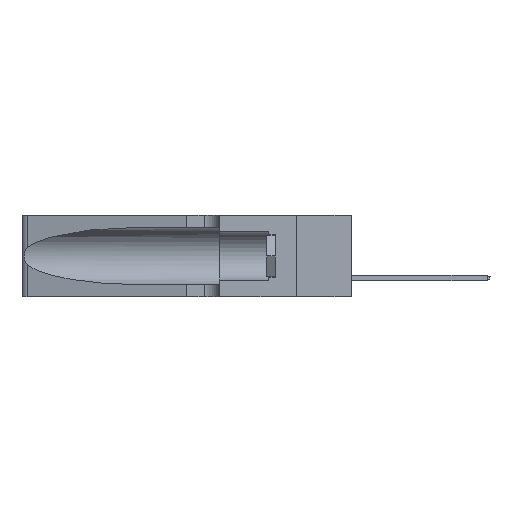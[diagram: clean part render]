
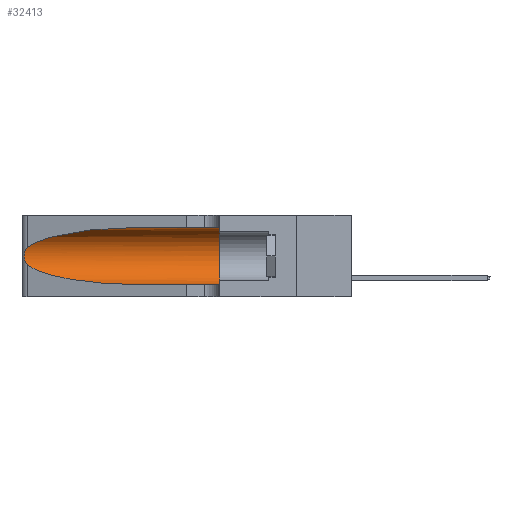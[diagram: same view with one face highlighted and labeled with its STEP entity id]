
A CAD part, left-side view. The second image highlights one B-rep face of the part: STEP entity #32413.
In plain terms, the highlighted cylindrical face has radius 3.308 mm (diameter 6.617 mm), a partial arc.
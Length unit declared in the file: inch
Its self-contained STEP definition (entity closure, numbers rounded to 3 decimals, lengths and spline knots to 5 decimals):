
#82 = CIRCLE ( 'NONE', #31931, 0.13025 ) ;
#206 = VERTEX_POINT ( 'NONE', #14454 ) ;
#1051 = DIRECTION ( 'NONE',  ( 0., -1., 0. ) ) ;
#1223 = CARTESIAN_POINT ( 'NONE',  ( 0.25487, 1.22718, 0.14631 ) ) ;
#1243 = CARTESIAN_POINT ( 'NONE',  ( 0.26075, 1.23896, 0.19203 ) ) ;
#1700 = ORIENTED_EDGE ( 'NONE', *, *, #35580, .T. ) ;
#3316 = EDGE_CURVE ( 'NONE', #7978, #206, #35586, .T. ) ;
#3819 = LINE ( 'NONE', #14539, #11201 ) ;
#4359 = EDGE_CURVE ( 'NONE', #7978, #28881, #15083, .T. ) ;
#5092 = CARTESIAN_POINT ( 'NONE',  ( 0.25856, 1.23593, 0.16098 ) ) ;
#5230 = CARTESIAN_POINT ( 'NONE',  ( 0.1305, 0.72297, 0.31525 ) ) ;
#6283 = CARTESIAN_POINT ( 'NONE',  ( 0.2373, 1.15595, 0.28018 ) ) ;
#6428 = CARTESIAN_POINT ( 'NONE',  ( 0.1305, 0.72297, 0.31525 ) ) ;
#7680 = CARTESIAN_POINT ( 'NONE',  ( 0.1305, 1.61858, 0.185 ) ) ;
#7978 = VERTEX_POINT ( 'NONE', #5230 ) ;
#8002 = CARTESIAN_POINT ( 'NONE',  ( 0.26017, 1.23833, 0.17102 ) ) ;
#8470 = CARTESIAN_POINT ( 'NONE',  ( 0.25487, 1.22718, 0.22369 ) ) ;
#9814 = CARTESIAN_POINT ( 'NONE',  ( 0.1305, 0.35, 0.185 ) ) ;
#10583 = CARTESIAN_POINT ( 'NONE',  ( 0.1305, 0.35, 0.31525 ) ) ;
#10893 = CARTESIAN_POINT ( 'NONE',  ( 0.18966, 0.96281, 0.05475 ) ) ;
#11041 = CARTESIAN_POINT ( 'NONE',  ( 0.1305, 0.72297, 0.05475 ) ) ;
#11070 = CARTESIAN_POINT ( 'NONE',  ( 0.1305, 0.35, 0.05475 ) ) ;
#11201 = VECTOR ( 'NONE', #21382, 39.37008 ) ;
#11645 = ORIENTED_EDGE ( 'NONE', *, *, #4359, .F. ) ;
#12899 = DIRECTION ( 'NONE',  ( 0., 1., 0. ) ) ;
#13308 = CARTESIAN_POINT ( 'NONE',  ( 0.18966, 0.96281, 0.31525 ) ) ;
#13365 = CARTESIAN_POINT ( 'NONE',  ( 0.1305, 0.72297, 0.05475 ) ) ;
#13626 = CARTESIAN_POINT ( 'NONE',  ( 0.1305, 1.61858, 0.31525 ) ) ;
#13646 = EDGE_CURVE ( 'NONE', #206, #31833, #38542, .T. ) ;
#14454 = CARTESIAN_POINT ( 'NONE',  ( 0.25487, 1.22718, 0.22369 ) ) ;
#14539 = CARTESIAN_POINT ( 'NONE',  ( 0.1305, 1.61858, 0.05475 ) ) ;
#14597 = DIRECTION ( 'NONE',  ( 0., 0., -1. ) ) ;
#15083 = LINE ( 'NONE', #13626, #16662 ) ;
#15721 = CYLINDRICAL_SURFACE ( 'NONE', #19944, 0.13025 ) ;
#16662 = VECTOR ( 'NONE', #27362, 39.37008 ) ;
#17734 = EDGE_CURVE ( 'NONE', #28881, #19556, #82, .T. ) ;
#18363 = CARTESIAN_POINT ( 'NONE',  ( 0.25639, 1.23184, 0.21858 ) ) ;
#19556 = VERTEX_POINT ( 'NONE', #11070 ) ;
#19944 = AXIS2_PLACEMENT_3D ( 'NONE', #7680, #1051, #14597 ) ;
#20816 = CARTESIAN_POINT ( 'NONE',  ( 0.2373, 1.15595, 0.08982 ) ) ;
#21382 = DIRECTION ( 'NONE',  ( 0., -1., 0. ) ) ;
#21464 = CARTESIAN_POINT ( 'NONE',  ( 0.26075, 1.23896, 0.178 ) ) ;
#21618 = CARTESIAN_POINT ( 'NONE',  ( 0.25854, 1.2359, 0.20912 ) ) ;
#25204 = ORIENTED_EDGE ( 'NONE', *, *, #3316, .T. ) ;
#25352 = CARTESIAN_POINT ( 'NONE',  ( 0.25555, 1.22994, 0.2215 ) ) ;
#26690 = VERTEX_POINT ( 'NONE', #13365 ) ;
#27362 = DIRECTION ( 'NONE',  ( 0., -1., 0. ) ) ;
#28578 = CARTESIAN_POINT ( 'NONE',  ( 0.25555, 1.22993, 0.14849 ) ) ;
#28733 = CARTESIAN_POINT ( 'NONE',  ( 0.25639, 1.23186, 0.15144 ) ) ;
#28881 = VERTEX_POINT ( 'NONE', #10583 ) ;
#29905 = CARTESIAN_POINT ( 'NONE',  ( 0.25487, 1.22718, 0.22369 ) ) ;
#30506 = ORIENTED_EDGE ( 'NONE', *, *, #37550, .T. ) ;
#31833 = VERTEX_POINT ( 'NONE', #1223 ) ;
#31931 = AXIS2_PLACEMENT_3D ( 'NONE', #9814, #12899, #33477 ) ;
#32413 = ADVANCED_FACE ( 'NONE', ( #40983 ), #15721, .F. ) ;
#33477 = DIRECTION ( 'NONE',  ( 0., 0., 1. ) ) ;
#33951 = EDGE_LOOP ( 'NONE', ( #25204, #42934, #30506, #1700, #38205, #11645 ) ) ;
#34268 = CARTESIAN_POINT ( 'NONE',  ( 0.25487, 1.22718, 0.14631 ) ) ;
#35039 = CARTESIAN_POINT ( 'NONE',  ( 0.25789, 1.23486, 0.15765 ) ) ;
#35580 = EDGE_CURVE ( 'NONE', #26690, #19556, #3819, .T. ) ;
#35586 =( BOUNDED_CURVE ( )  B_SPLINE_CURVE ( 3, ( #6428, #13308, #6283, #29905 ),
 .UNSPECIFIED., .F., .F. ) 
 B_SPLINE_CURVE_WITH_KNOTS ( ( 4, 4 ),
 ( 1.5708, 2.84003 ),
 .UNSPECIFIED. ) 
 CURVE ( )  GEOMETRIC_REPRESENTATION_ITEM ( )  RATIONAL_B_SPLINE_CURVE ( ( 1., 0.87, 0.87, 1. ) ) 
 REPRESENTATION_ITEM ( '' )  );
#37550 = EDGE_CURVE ( 'NONE', #31833, #26690, #43675, .T. ) ;
#38205 = ORIENTED_EDGE ( 'NONE', *, *, #17734, .F. ) ;
#38445 = CARTESIAN_POINT ( 'NONE',  ( 0.25487, 1.22718, 0.14631 ) ) ;
#38542 = B_SPLINE_CURVE_WITH_KNOTS ( 'NONE', 3,
 ( #8470, #25352, #18363, #41963, #21618, #41650, #1243, #21464, #8002, #5092, #35039, #28733, #28578, #38445 ),
 .UNSPECIFIED., .F., .F.,
 ( 4, 2, 2, 2, 2, 2, 4 ),
 ( 0., 0.00027, 0.00053, 0.00107, 0.0016, 0.00187, 0.00214 ),
 .UNSPECIFIED. ) ;
#40983 = FACE_OUTER_BOUND ( 'NONE', #33951, .T. ) ;
#41650 = CARTESIAN_POINT ( 'NONE',  ( 0.26018, 1.23835, 0.19895 ) ) ;
#41963 = CARTESIAN_POINT ( 'NONE',  ( 0.25787, 1.23484, 0.2124 ) ) ;
#42934 = ORIENTED_EDGE ( 'NONE', *, *, #13646, .T. ) ;
#43675 =( BOUNDED_CURVE ( )  B_SPLINE_CURVE ( 3, ( #34268, #20816, #10893, #11041 ),
 .UNSPECIFIED., .F., .F. ) 
 B_SPLINE_CURVE_WITH_KNOTS ( ( 4, 4 ),
 ( 3.44316, 4.71239 ),
 .UNSPECIFIED. ) 
 CURVE ( )  GEOMETRIC_REPRESENTATION_ITEM ( )  RATIONAL_B_SPLINE_CURVE ( ( 1., 0.87, 0.87, 1. ) ) 
 REPRESENTATION_ITEM ( '' )  );
